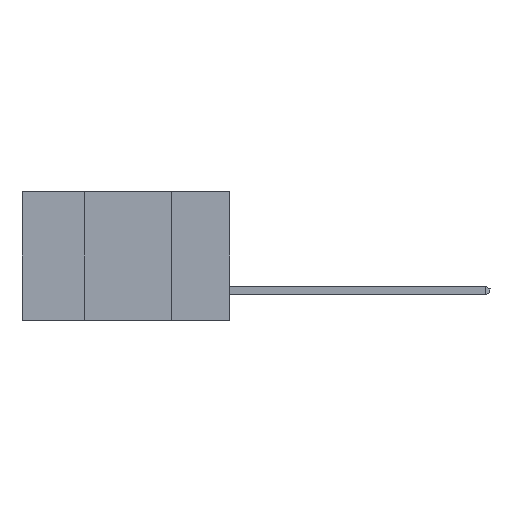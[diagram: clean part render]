
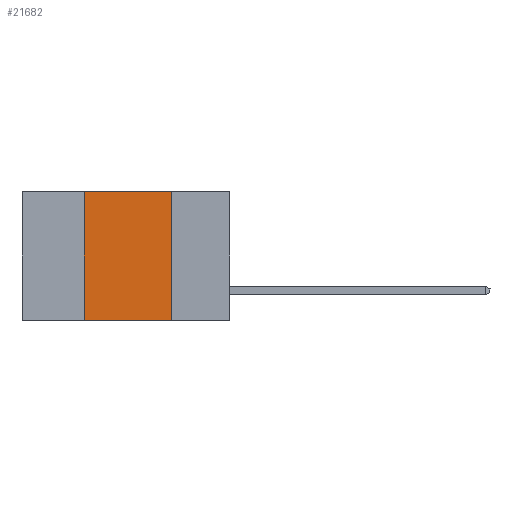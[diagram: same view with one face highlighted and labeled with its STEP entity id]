
A CAD part, left-side view. The second image highlights one B-rep face of the part: STEP entity #21682.
In plain terms, the highlighted planar face has unit normal (-1, 0, 0).
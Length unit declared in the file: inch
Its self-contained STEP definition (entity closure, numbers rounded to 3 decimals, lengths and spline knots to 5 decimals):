
#2072 = LINE ( 'NONE', #18251, #4642 ) ;
#2435 = CARTESIAN_POINT ( 'NONE',  ( 0., 0.17, -0.37 ) ) ;
#2660 = LINE ( 'NONE', #2435, #16913 ) ;
#2800 = EDGE_CURVE ( 'NONE', #9146, #6445, #2072, .T. ) ;
#4260 = CARTESIAN_POINT ( 'NONE',  ( 0., 0.6, -0.37 ) ) ;
#4642 = VECTOR ( 'NONE', #6184, 39.37008 ) ;
#5985 = LINE ( 'NONE', #4260, #15101 ) ;
#6184 = DIRECTION ( 'NONE',  ( 0., 0., 1. ) ) ;
#6191 = ORIENTED_EDGE ( 'NONE', *, *, #8061, .T. ) ;
#6445 = VERTEX_POINT ( 'NONE', #13268 ) ;
#7274 = DIRECTION ( 'NONE',  ( 0., 0., -1. ) ) ;
#7600 = DIRECTION ( 'NONE',  ( 0., 0., -1. ) ) ;
#8061 = EDGE_CURVE ( 'NONE', #9146, #13711, #5985, .T. ) ;
#8258 = CARTESIAN_POINT ( 'NONE',  ( 0., 0.42, -0.37 ) ) ;
#8469 = ORIENTED_EDGE ( 'NONE', *, *, #15841, .F. ) ;
#8891 = CARTESIAN_POINT ( 'NONE',  ( 0., 0.6, 0. ) ) ;
#9146 = VERTEX_POINT ( 'NONE', #8258 ) ;
#9213 = AXIS2_PLACEMENT_3D ( 'NONE', #8891, #19574, #7274 ) ;
#10280 = VERTEX_POINT ( 'NONE', #14511 ) ;
#10619 = FACE_OUTER_BOUND ( 'NONE', #10791, .T. ) ;
#10791 = EDGE_LOOP ( 'NONE', ( #12171, #8469, #22570, #6191 ) ) ;
#11355 = LINE ( 'NONE', #20083, #12011 ) ;
#12011 = VECTOR ( 'NONE', #13419, 39.37008 ) ;
#12171 = ORIENTED_EDGE ( 'NONE', *, *, #20584, .F. ) ;
#12202 = CARTESIAN_POINT ( 'NONE',  ( 0., 0.17, -0.37 ) ) ;
#13268 = CARTESIAN_POINT ( 'NONE',  ( 0., 0.42, 0. ) ) ;
#13419 = DIRECTION ( 'NONE',  ( 0., -1., 0. ) ) ;
#13711 = VERTEX_POINT ( 'NONE', #12202 ) ;
#14511 = CARTESIAN_POINT ( 'NONE',  ( 0., 0.17, 0. ) ) ;
#15101 = VECTOR ( 'NONE', #18283, 39.37008 ) ;
#15841 = EDGE_CURVE ( 'NONE', #6445, #10280, #11355, .T. ) ;
#16913 = VECTOR ( 'NONE', #7600, 39.37008 ) ;
#17494 = PLANE ( 'NONE',  #9213 ) ;
#18251 = CARTESIAN_POINT ( 'NONE',  ( 0., 0.42, -0.37 ) ) ;
#18283 = DIRECTION ( 'NONE',  ( 0., -1., 0. ) ) ;
#19574 = DIRECTION ( 'NONE',  ( 1., 0., 0. ) ) ;
#20083 = CARTESIAN_POINT ( 'NONE',  ( 0., 0.6, 0. ) ) ;
#20584 = EDGE_CURVE ( 'NONE', #10280, #13711, #2660, .T. ) ;
#21682 = ADVANCED_FACE ( 'NONE', ( #10619 ), #17494, .F. ) ;
#22570 = ORIENTED_EDGE ( 'NONE', *, *, #2800, .F. ) ;
